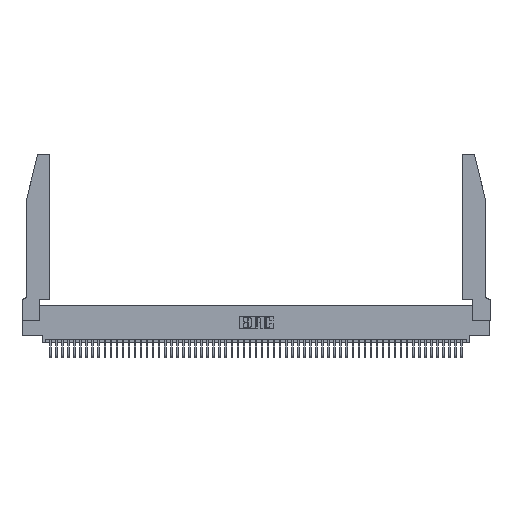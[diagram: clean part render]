
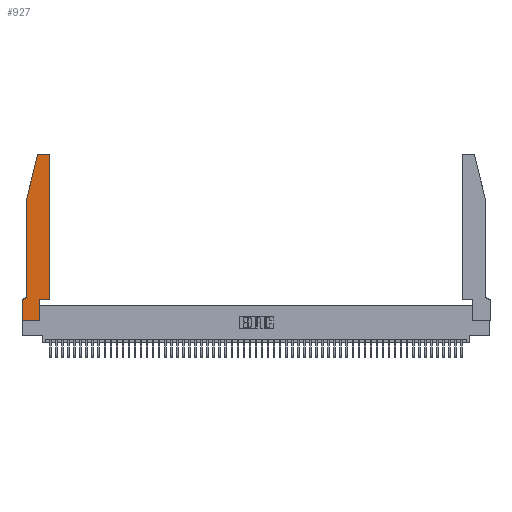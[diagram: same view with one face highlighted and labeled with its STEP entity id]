
A CAD part, top view. The second image highlights one B-rep face of the part: STEP entity #927.
In plain terms, the highlighted planar face has unit normal (0, 0, 1).
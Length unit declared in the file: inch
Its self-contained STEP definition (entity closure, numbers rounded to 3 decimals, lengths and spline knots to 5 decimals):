
#290 = EDGE_CURVE ( 'NONE', #22576, #4365, #42033, .T. ) ;
#302 = EDGE_CURVE ( 'NONE', #35240, #28347, #31143, .T. ) ;
#927 = ADVANCED_FACE ( 'NONE', ( #22033 ), #1890, .T. ) ;
#1019 = EDGE_LOOP ( 'NONE', ( #26873, #16876, #50070, #47767, #30472, #27523, #7794, #28619, #22454, #23139, #8859, #21189 ) ) ;
#1571 = CARTESIAN_POINT ( 'NONE',  ( 0.0755, 2., 0.37 ) ) ;
#1890 = PLANE ( 'NONE',  #3789 ) ;
#2099 = EDGE_CURVE ( 'NONE', #7568, #32841, #34558, .T. ) ;
#2297 = VERTEX_POINT ( 'NONE', #52064 ) ;
#2975 = VERTEX_POINT ( 'NONE', #7102 ) ;
#3205 = CARTESIAN_POINT ( 'NONE',  ( 0.25487, 2.72718, 0.37 ) ) ;
#3464 = LINE ( 'NONE', #19584, #16943 ) ;
#3700 = EDGE_CURVE ( 'NONE', #28347, #19677, #3464, .T. ) ;
#3715 = CARTESIAN_POINT ( 'NONE',  ( 0.4505, 0.35, 0.37 ) ) ;
#3789 = AXIS2_PLACEMENT_3D ( 'NONE', #14274, #18404, #47172 ) ;
#4365 = VERTEX_POINT ( 'NONE', #3715 ) ;
#4480 = DIRECTION ( 'NONE',  ( 0., 0., -1. ) ) ;
#5738 = LINE ( 'NONE', #40608, #37235 ) ;
#5743 = DIRECTION ( 'NONE',  ( 0., -1., 0. ) ) ;
#5839 = AXIS2_PLACEMENT_3D ( 'NONE', #18654, #47415, #22803 ) ;
#7102 = CARTESIAN_POINT ( 'NONE',  ( 0., 0.35, 0.37 ) ) ;
#7568 = VERTEX_POINT ( 'NONE', #24311 ) ;
#7794 = ORIENTED_EDGE ( 'NONE', *, *, #14056, .T. ) ;
#7919 = CARTESIAN_POINT ( 'NONE',  ( 0.284, 2.72, 0.37 ) ) ;
#8783 = CARTESIAN_POINT ( 'NONE',  ( 0.0055, 0.35, 0.37 ) ) ;
#8859 = ORIENTED_EDGE ( 'NONE', *, *, #44868, .T. ) ;
#9148 = LINE ( 'NONE', #16493, #52858 ) ;
#12017 = DIRECTION ( 'NONE',  ( 1., 0., 0. ) ) ;
#12138 = EDGE_CURVE ( 'NONE', #2297, #22576, #5738, .T. ) ;
#12588 = VECTOR ( 'NONE', #5743, 39.37008 ) ;
#12695 = AXIS2_PLACEMENT_3D ( 'NONE', #7919, #36699, #12017 ) ;
#13246 = VERTEX_POINT ( 'NONE', #8783 ) ;
#14056 = EDGE_CURVE ( 'NONE', #2975, #51255, #15875, .T. ) ;
#14274 = CARTESIAN_POINT ( 'NONE',  ( 0., 0.35, 0.37 ) ) ;
#15758 = CARTESIAN_POINT ( 'NONE',  ( 0., 0., 0.37 ) ) ;
#15806 = CARTESIAN_POINT ( 'NONE',  ( 0.2865, 0.35, 0.37 ) ) ;
#15875 = LINE ( 'NONE', #42139, #37205 ) ;
#16493 = CARTESIAN_POINT ( 'NONE',  ( 0., 0., 0.37 ) ) ;
#16796 = VECTOR ( 'NONE', #23702, 39.37008 ) ;
#16876 = ORIENTED_EDGE ( 'NONE', *, *, #45832, .T. ) ;
#16943 = VECTOR ( 'NONE', #44210, 39.37008 ) ;
#18186 = CARTESIAN_POINT ( 'NONE',  ( 0.284, 2.75, 0.37 ) ) ;
#18404 = DIRECTION ( 'NONE',  ( 0., 0., 1. ) ) ;
#18654 = CARTESIAN_POINT ( 'NONE',  ( 0.4205, 2.72, 0.37 ) ) ;
#18692 = LINE ( 'NONE', #46799, #20002 ) ;
#18716 = EDGE_CURVE ( 'NONE', #38073, #7568, #26409, .T. ) ;
#19219 = CIRCLE ( 'NONE', #32063, 0.07 ) ;
#19584 = CARTESIAN_POINT ( 'NONE',  ( 0.2605, 2.75, 0.37 ) ) ;
#19677 = VERTEX_POINT ( 'NONE', #18186 ) ;
#20002 = VECTOR ( 'NONE', #26365, 39.37008 ) ;
#21189 = ORIENTED_EDGE ( 'NONE', *, *, #302, .T. ) ;
#21648 = DIRECTION ( 'NONE',  ( 0., -1., 0. ) ) ;
#22033 = FACE_OUTER_BOUND ( 'NONE', #1019, .T. ) ;
#22454 = ORIENTED_EDGE ( 'NONE', *, *, #12138, .T. ) ;
#22576 = VERTEX_POINT ( 'NONE', #15806 ) ;
#22651 = CARTESIAN_POINT ( 'NONE',  ( 0.4505, 2.72, 0.37 ) ) ;
#22803 = DIRECTION ( 'NONE',  ( 1., 0., 0. ) ) ;
#23139 = ORIENTED_EDGE ( 'NONE', *, *, #290, .T. ) ;
#23702 = DIRECTION ( 'NONE',  ( -1., 0., 0. ) ) ;
#24311 = CARTESIAN_POINT ( 'NONE',  ( 0.0755, 2., 0.37 ) ) ;
#24398 = CIRCLE ( 'NONE', #12695, 0.03 ) ;
#24644 = EDGE_CURVE ( 'NONE', #51255, #2297, #9148, .T. ) ;
#26365 = DIRECTION ( 'NONE',  ( 0., 1., 0. ) ) ;
#26409 = LINE ( 'NONE', #49739, #36064 ) ;
#26804 = DIRECTION ( 'NONE',  ( 1., 0., 0. ) ) ;
#26873 = ORIENTED_EDGE ( 'NONE', *, *, #3700, .T. ) ;
#27523 = ORIENTED_EDGE ( 'NONE', *, *, #38069, .T. ) ;
#28347 = VERTEX_POINT ( 'NONE', #41889 ) ;
#28619 = ORIENTED_EDGE ( 'NONE', *, *, #24644, .T. ) ;
#29109 = CARTESIAN_POINT ( 'NONE',  ( 0.0055, 0.42, 0.37 ) ) ;
#29291 = DIRECTION ( 'NONE',  ( -0.239, -0.971, 0. ) ) ;
#30472 = ORIENTED_EDGE ( 'NONE', *, *, #45939, .T. ) ;
#31143 = CIRCLE ( 'NONE', #5839, 0.03 ) ;
#32063 = AXIS2_PLACEMENT_3D ( 'NONE', #29109, #4480, #33262 ) ;
#32428 = VECTOR ( 'NONE', #26804, 39.37008 ) ;
#32841 = VERTEX_POINT ( 'NONE', #43770 ) ;
#33262 = DIRECTION ( 'NONE',  ( -1., 0., 0. ) ) ;
#34558 = LINE ( 'NONE', #1571, #12588 ) ;
#35240 = VERTEX_POINT ( 'NONE', #22651 ) ;
#36064 = VECTOR ( 'NONE', #29291, 39.37008 ) ;
#36527 = DIRECTION ( 'NONE',  ( 0., 1., 0. ) ) ;
#36699 = DIRECTION ( 'NONE',  ( 0., 0., 1. ) ) ;
#37205 = VECTOR ( 'NONE', #21648, 39.37008 ) ;
#37235 = VECTOR ( 'NONE', #36527, 39.37008 ) ;
#38069 = EDGE_CURVE ( 'NONE', #13246, #2975, #38684, .T. ) ;
#38073 = VERTEX_POINT ( 'NONE', #3205 ) ;
#38684 = LINE ( 'NONE', #52422, #16796 ) ;
#40608 = CARTESIAN_POINT ( 'NONE',  ( 0.2865, 0.35, 0.37 ) ) ;
#41889 = CARTESIAN_POINT ( 'NONE',  ( 0.4205, 2.75, 0.37 ) ) ;
#42033 = LINE ( 'NONE', #51360, #32428 ) ;
#42139 = CARTESIAN_POINT ( 'NONE',  ( 0., 0., 0.37 ) ) ;
#43770 = CARTESIAN_POINT ( 'NONE',  ( 0.0755, 0.42, 0.37 ) ) ;
#44210 = DIRECTION ( 'NONE',  ( -1., 0., 0. ) ) ;
#44868 = EDGE_CURVE ( 'NONE', #4365, #35240, #18692, .T. ) ;
#45832 = EDGE_CURVE ( 'NONE', #19677, #38073, #24398, .T. ) ;
#45939 = EDGE_CURVE ( 'NONE', #32841, #13246, #19219, .T. ) ;
#46799 = CARTESIAN_POINT ( 'NONE',  ( 0.4505, 0.35, 0.37 ) ) ;
#47172 = DIRECTION ( 'NONE',  ( 1., 0., 0. ) ) ;
#47415 = DIRECTION ( 'NONE',  ( 0., 0., 1. ) ) ;
#47767 = ORIENTED_EDGE ( 'NONE', *, *, #2099, .T. ) ;
#49383 = DIRECTION ( 'NONE',  ( 1., 0., 0. ) ) ;
#49739 = CARTESIAN_POINT ( 'NONE',  ( 0.0755, 2., 0.37 ) ) ;
#50070 = ORIENTED_EDGE ( 'NONE', *, *, #18716, .T. ) ;
#51255 = VERTEX_POINT ( 'NONE', #15758 ) ;
#51360 = CARTESIAN_POINT ( 'NONE',  ( 0.4505, 0.35, 0.37 ) ) ;
#52064 = CARTESIAN_POINT ( 'NONE',  ( 0.2865, 0., 0.37 ) ) ;
#52422 = CARTESIAN_POINT ( 'NONE',  ( 0.0755, 0.35, 0.37 ) ) ;
#52858 = VECTOR ( 'NONE', #49383, 39.37008 ) ;
